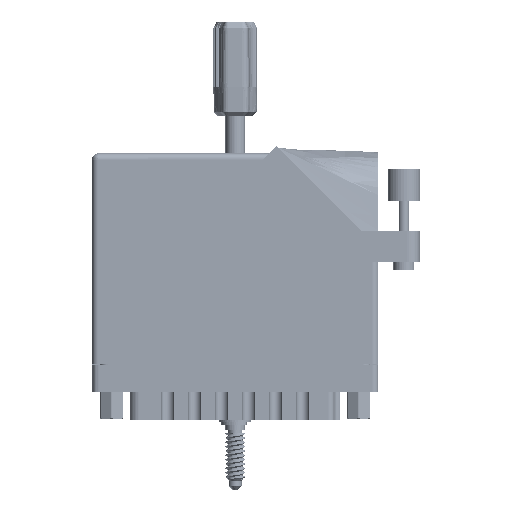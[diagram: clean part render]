
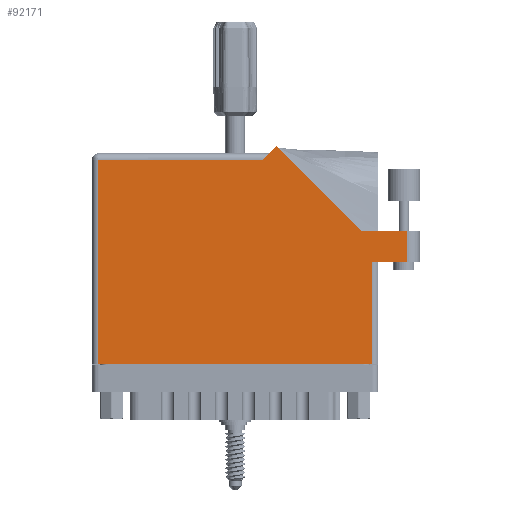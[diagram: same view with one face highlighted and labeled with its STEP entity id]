
A CAD part, front view. The second image highlights one B-rep face of the part: STEP entity #92171.
In plain terms, the highlighted face is planar.
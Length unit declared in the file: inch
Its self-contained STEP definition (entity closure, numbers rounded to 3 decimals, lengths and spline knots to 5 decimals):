
#1726 = EDGE_CURVE ( 'NONE', #84721, #56759, #103815, .T. ) ;
#2773 = LINE ( 'NONE', #76102, #50304 ) ;
#5946 = VECTOR ( 'NONE', #12549, 39.37008 ) ;
#8160 = EDGE_CURVE ( 'NONE', #46048, #15036, #32139, .T. ) ;
#9763 = VECTOR ( 'NONE', #107085, 39.37008 ) ;
#12242 = EDGE_CURVE ( 'NONE', #89278, #105099, #19762, .T. ) ;
#12549 = DIRECTION ( 'NONE',  ( -1., 0., 0. ) ) ;
#12758 = ORIENTED_EDGE ( 'NONE', *, *, #107873, .T. ) ;
#13968 = VERTEX_POINT ( 'NONE', #38628 ) ;
#15036 = VERTEX_POINT ( 'NONE', #54046 ) ;
#16604 = ORIENTED_EDGE ( 'NONE', *, *, #35370, .T. ) ;
#16909 = DIRECTION ( 'NONE',  ( -1., 0., 0. ) ) ;
#19762 = LINE ( 'NONE', #115132, #9763 ) ;
#21359 = LINE ( 'NONE', #81239, #70298 ) ;
#23106 = CARTESIAN_POINT ( 'NONE',  ( 3.03, 1.287, 0. ) ) ;
#24746 = DIRECTION ( 'NONE',  ( 1., 0., 0. ) ) ;
#26322 = VECTOR ( 'NONE', #64982, 39.37008 ) ;
#27776 = DIRECTION ( 'NONE',  ( 0., 0., -1. ) ) ;
#29092 = VECTOR ( 'NONE', #71041, 39.37008 ) ;
#32139 = LINE ( 'NONE', #92343, #26322 ) ;
#32961 = EDGE_CURVE ( 'NONE', #79562, #87051, #21359, .T. ) ;
#33701 = VECTOR ( 'NONE', #55089, 39.37008 ) ;
#35370 = EDGE_CURVE ( 'NONE', #56759, #13968, #58118, .T. ) ;
#35394 = VECTOR ( 'NONE', #24746, 39.37008 ) ;
#38628 = CARTESIAN_POINT ( 'NONE',  ( 0.062, 0., 0. ) ) ;
#45410 = PLANE ( 'NONE',  #52647 ) ;
#45822 = CARTESIAN_POINT ( 'NONE',  ( 0.062, 0., 0. ) ) ;
#46048 = VERTEX_POINT ( 'NONE', #90734 ) ;
#48236 = CARTESIAN_POINT ( 'NONE',  ( 1.643, 1.968, 0. ) ) ;
#50304 = VECTOR ( 'NONE', #94190, 39.37008 ) ;
#52647 = AXIS2_PLACEMENT_3D ( 'NONE', #109026, #27776, #16909 ) ;
#53517 = LINE ( 'NONE', #70243, #29092 ) ;
#54046 = CARTESIAN_POINT ( 'NONE',  ( 1.77571, 2.10071, 0. ) ) ;
#55089 = DIRECTION ( 'NONE',  ( 0., -1., 0. ) ) ;
#56261 = FACE_OUTER_BOUND ( 'NONE', #74604, .T. ) ;
#56759 = VERTEX_POINT ( 'NONE', #95400 ) ;
#58118 = LINE ( 'NONE', #45822, #33701 ) ;
#59198 = LINE ( 'NONE', #67221, #73606 ) ;
#62184 = EDGE_CURVE ( 'NONE', #87051, #89278, #53517, .T. ) ;
#62523 = EDGE_CURVE ( 'NONE', #105099, #46048, #59198, .T. ) ;
#63632 = EDGE_CURVE ( 'NONE', #15036, #84721, #2773, .T. ) ;
#64982 = DIRECTION ( 'NONE',  ( -0.707, 0.707, 0. ) ) ;
#67221 = CARTESIAN_POINT ( 'NONE',  ( 3.155, 1.287, 0. ) ) ;
#70243 = CARTESIAN_POINT ( 'NONE',  ( 2.755, 0.98, 0. ) ) ;
#70298 = VECTOR ( 'NONE', #80857, 39.37008 ) ;
#71041 = DIRECTION ( 'NONE',  ( 1., 0., 0. ) ) ;
#71955 = ORIENTED_EDGE ( 'NONE', *, *, #32961, .T. ) ;
#73606 = VECTOR ( 'NONE', #84538, 39.37008 ) ;
#74604 = EDGE_LOOP ( 'NONE', ( #111517, #101880, #102375, #97811, #90951, #101963, #16604, #12758, #71955 ) ) ;
#76073 = CARTESIAN_POINT ( 'NONE',  ( 0., 1.968, 0. ) ) ;
#76102 = CARTESIAN_POINT ( 'NONE',  ( 1.705, 2.03, 0. ) ) ;
#79562 = VERTEX_POINT ( 'NONE', #89799 ) ;
#80857 = DIRECTION ( 'NONE',  ( 0., 1., 0. ) ) ;
#81239 = CARTESIAN_POINT ( 'NONE',  ( 2.693, 0.98, 0. ) ) ;
#84538 = DIRECTION ( 'NONE',  ( -1., 0., 0. ) ) ;
#84721 = VERTEX_POINT ( 'NONE', #48236 ) ;
#87051 = VERTEX_POINT ( 'NONE', #115020 ) ;
#89278 = VERTEX_POINT ( 'NONE', #105866 ) ;
#89799 = CARTESIAN_POINT ( 'NONE',  ( 2.693, 0., 0. ) ) ;
#90734 = CARTESIAN_POINT ( 'NONE',  ( 2.58942, 1.287, 0. ) ) ;
#90951 = ORIENTED_EDGE ( 'NONE', *, *, #63632, .T. ) ;
#92171 = ADVANCED_FACE ( 'NONE', ( #56261 ), #45410, .F. ) ;
#92343 = CARTESIAN_POINT ( 'NONE',  ( 2.58942, 1.287, 0. ) ) ;
#94190 = DIRECTION ( 'NONE',  ( -0.707, -0.707, 0. ) ) ;
#95400 = CARTESIAN_POINT ( 'NONE',  ( 0.062, 1.968, 0. ) ) ;
#97573 = CARTESIAN_POINT ( 'NONE',  ( 0., 0., 0. ) ) ;
#97811 = ORIENTED_EDGE ( 'NONE', *, *, #8160, .T. ) ;
#101880 = ORIENTED_EDGE ( 'NONE', *, *, #12242, .T. ) ;
#101963 = ORIENTED_EDGE ( 'NONE', *, *, #1726, .T. ) ;
#102375 = ORIENTED_EDGE ( 'NONE', *, *, #62523, .T. ) ;
#103815 = LINE ( 'NONE', #76073, #5946 ) ;
#105099 = VERTEX_POINT ( 'NONE', #23106 ) ;
#105866 = CARTESIAN_POINT ( 'NONE',  ( 3.03, 0.98, 0. ) ) ;
#105950 = LINE ( 'NONE', #97573, #35394 ) ;
#107085 = DIRECTION ( 'NONE',  ( 0., 1., 0. ) ) ;
#107873 = EDGE_CURVE ( 'NONE', #13968, #79562, #105950, .T. ) ;
#109026 = CARTESIAN_POINT ( 'NONE',  ( 0., 2.03, 0. ) ) ;
#111517 = ORIENTED_EDGE ( 'NONE', *, *, #62184, .T. ) ;
#115020 = CARTESIAN_POINT ( 'NONE',  ( 2.693, 0.98, 0. ) ) ;
#115132 = CARTESIAN_POINT ( 'NONE',  ( 3.03, 1.287, 0. ) ) ;
